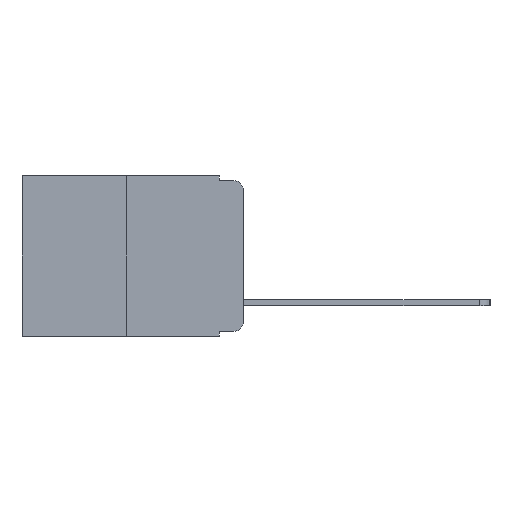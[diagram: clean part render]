
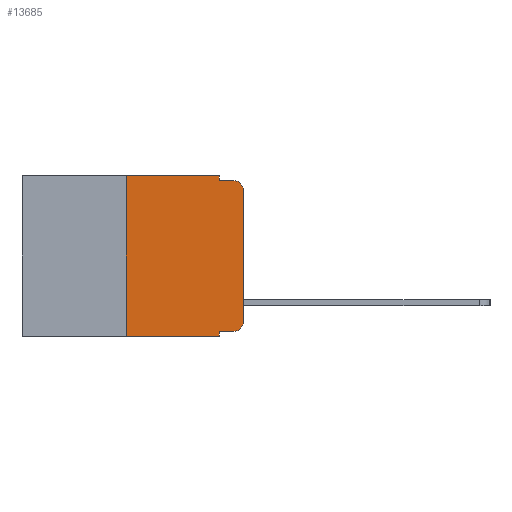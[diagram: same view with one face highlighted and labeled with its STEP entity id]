
A CAD part, left-side view. The second image highlights one B-rep face of the part: STEP entity #13685.
In plain terms, the highlighted planar face has unit normal (-1, 0, 0).
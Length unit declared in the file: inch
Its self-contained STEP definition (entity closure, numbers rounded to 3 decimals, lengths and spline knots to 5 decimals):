
#5 = DIRECTION ( 'NONE',  ( -1., 0., 0. ) ) ;
#22 = VERTEX_POINT ( 'NONE', #6752 ) ;
#108 = DIRECTION ( 'NONE',  ( 0., -1., 0. ) ) ;
#171 = CARTESIAN_POINT ( 'NONE',  ( 0., 0.02, -0.333 ) ) ;
#182 = VECTOR ( 'NONE', #1025, 39.37008 ) ;
#249 = DIRECTION ( 'NONE',  ( 0., -1., 0. ) ) ;
#274 = DIRECTION ( 'NONE',  ( 0., 0., 1. ) ) ;
#544 = VERTEX_POINT ( 'NONE', #7905 ) ;
#716 = ORIENTED_EDGE ( 'NONE', *, *, #8740, .F. ) ;
#798 = VERTEX_POINT ( 'NONE', #12643 ) ;
#1025 = DIRECTION ( 'NONE',  ( 0., 0., -1. ) ) ;
#1288 = CIRCLE ( 'NONE', #3294, 0.02 ) ;
#1515 = PLANE ( 'NONE',  #12511 ) ;
#1677 = CARTESIAN_POINT ( 'NONE',  ( 0., 0.051, -0.01 ) ) ;
#1832 = EDGE_CURVE ( 'NONE', #22, #4384, #10424, .T. ) ;
#2120 = VECTOR ( 'NONE', #6330, 39.37008 ) ;
#2640 = LINE ( 'NONE', #17333, #18542 ) ;
#2920 = CARTESIAN_POINT ( 'NONE',  ( 0., 0.25, 0. ) ) ;
#3098 = DIRECTION ( 'NONE',  ( 0., 0., -1. ) ) ;
#3193 = LINE ( 'NONE', #6419, #19072 ) ;
#3294 = AXIS2_PLACEMENT_3D ( 'NONE', #9456, #5, #11020 ) ;
#4299 = EDGE_CURVE ( 'NONE', #798, #544, #13375, .T. ) ;
#4384 = VERTEX_POINT ( 'NONE', #14278 ) ;
#4403 = ORIENTED_EDGE ( 'NONE', *, *, #15636, .F. ) ;
#4504 = VECTOR ( 'NONE', #249, 39.37008 ) ;
#4765 = CARTESIAN_POINT ( 'NONE',  ( 0., 0., 0. ) ) ;
#5003 = VERTEX_POINT ( 'NONE', #2920 ) ;
#5086 = VERTEX_POINT ( 'NONE', #1677 ) ;
#5147 = VERTEX_POINT ( 'NONE', #12709 ) ;
#5205 = VECTOR ( 'NONE', #19713, 39.37008 ) ;
#5854 = AXIS2_PLACEMENT_3D ( 'NONE', #16201, #6972, #17721 ) ;
#6330 = DIRECTION ( 'NONE',  ( 0., 0., 1. ) ) ;
#6376 = CARTESIAN_POINT ( 'NONE',  ( 0., 0.051, 0. ) ) ;
#6419 = CARTESIAN_POINT ( 'NONE',  ( 0., 0.051, -0.01 ) ) ;
#6752 = CARTESIAN_POINT ( 'NONE',  ( 0., 0., -0.313 ) ) ;
#6857 = ORIENTED_EDGE ( 'NONE', *, *, #6937, .T. ) ;
#6921 = VERTEX_POINT ( 'NONE', #171 ) ;
#6937 = EDGE_CURVE ( 'NONE', #798, #6921, #12772, .T. ) ;
#6972 = DIRECTION ( 'NONE',  ( -1., 0., 0. ) ) ;
#7209 = FACE_OUTER_BOUND ( 'NONE', #7339, .T. ) ;
#7339 = EDGE_LOOP ( 'NONE', ( #19776, #8095, #4403, #12678, #716, #17207, #14109, #18604, #6857, #15066 ) ) ;
#7905 = CARTESIAN_POINT ( 'NONE',  ( 0., 0.051, -0.343 ) ) ;
#7979 = CARTESIAN_POINT ( 'NONE',  ( 0., 0.051, 0. ) ) ;
#8095 = ORIENTED_EDGE ( 'NONE', *, *, #14468, .T. ) ;
#8131 = CARTESIAN_POINT ( 'NONE',  ( 0., 0.051, -0.333 ) ) ;
#8185 = DIRECTION ( 'NONE',  ( 0., -1., 0. ) ) ;
#8386 = LINE ( 'NONE', #14300, #11998 ) ;
#8740 = EDGE_CURVE ( 'NONE', #5003, #16299, #8386, .T. ) ;
#9456 = CARTESIAN_POINT ( 'NONE',  ( 0., 0.02, -0.03 ) ) ;
#9565 = EDGE_CURVE ( 'NONE', #6921, #22, #16519, .T. ) ;
#10424 = LINE ( 'NONE', #4765, #2120 ) ;
#10447 = VERTEX_POINT ( 'NONE', #15479 ) ;
#10798 = CARTESIAN_POINT ( 'NONE',  ( 0., 0.473, 0. ) ) ;
#11020 = DIRECTION ( 'NONE',  ( 0., 0., -1. ) ) ;
#11998 = VECTOR ( 'NONE', #8185, 39.37008 ) ;
#12412 = DIRECTION ( 'NONE',  ( 1., 0., 0. ) ) ;
#12511 = AXIS2_PLACEMENT_3D ( 'NONE', #10798, #12412, #3098 ) ;
#12643 = CARTESIAN_POINT ( 'NONE',  ( 0., 0.051, -0.333 ) ) ;
#12678 = ORIENTED_EDGE ( 'NONE', *, *, #17812, .F. ) ;
#12709 = CARTESIAN_POINT ( 'NONE',  ( 0., 0.25, -0.343 ) ) ;
#12772 = LINE ( 'NONE', #8131, #4504 ) ;
#13375 = LINE ( 'NONE', #6376, #17417 ) ;
#13548 = CARTESIAN_POINT ( 'NONE',  ( 0., 0.051, 0. ) ) ;
#13685 = ADVANCED_FACE ( 'NONE', ( #7209 ), #1515, .F. ) ;
#14109 = ORIENTED_EDGE ( 'NONE', *, *, #16068, .T. ) ;
#14278 = CARTESIAN_POINT ( 'NONE',  ( 0., 0., -0.03 ) ) ;
#14300 = CARTESIAN_POINT ( 'NONE',  ( 0., 0.473, 0. ) ) ;
#14468 = EDGE_CURVE ( 'NONE', #4384, #10447, #1288, .T. ) ;
#15066 = ORIENTED_EDGE ( 'NONE', *, *, #9565, .T. ) ;
#15479 = CARTESIAN_POINT ( 'NONE',  ( 0., 0.02, -0.01 ) ) ;
#15613 = DIRECTION ( 'NONE',  ( 0., 0., -1. ) ) ;
#15636 = EDGE_CURVE ( 'NONE', #5086, #10447, #3193, .T. ) ;
#16068 = EDGE_CURVE ( 'NONE', #5147, #544, #17501, .T. ) ;
#16201 = CARTESIAN_POINT ( 'NONE',  ( 0., 0.02, -0.313 ) ) ;
#16266 = LINE ( 'NONE', #13548, #182 ) ;
#16299 = VERTEX_POINT ( 'NONE', #7979 ) ;
#16519 = CIRCLE ( 'NONE', #5854, 0.02 ) ;
#17207 = ORIENTED_EDGE ( 'NONE', *, *, #19322, .F. ) ;
#17333 = CARTESIAN_POINT ( 'NONE',  ( 0., 0.25, 0. ) ) ;
#17417 = VECTOR ( 'NONE', #15613, 39.37008 ) ;
#17501 = LINE ( 'NONE', #18207, #5205 ) ;
#17721 = DIRECTION ( 'NONE',  ( 0., 0., -1. ) ) ;
#17812 = EDGE_CURVE ( 'NONE', #16299, #5086, #16266, .T. ) ;
#18207 = CARTESIAN_POINT ( 'NONE',  ( 0., 0.473, -0.343 ) ) ;
#18542 = VECTOR ( 'NONE', #274, 39.37008 ) ;
#18604 = ORIENTED_EDGE ( 'NONE', *, *, #4299, .F. ) ;
#19072 = VECTOR ( 'NONE', #108, 39.37008 ) ;
#19322 = EDGE_CURVE ( 'NONE', #5147, #5003, #2640, .T. ) ;
#19713 = DIRECTION ( 'NONE',  ( 0., -1., 0. ) ) ;
#19776 = ORIENTED_EDGE ( 'NONE', *, *, #1832, .T. ) ;
